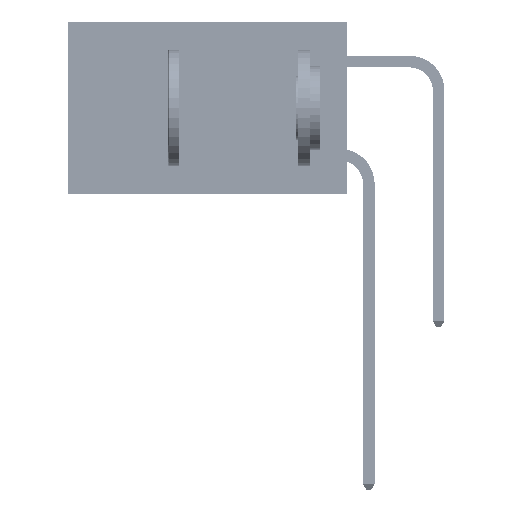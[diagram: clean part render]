
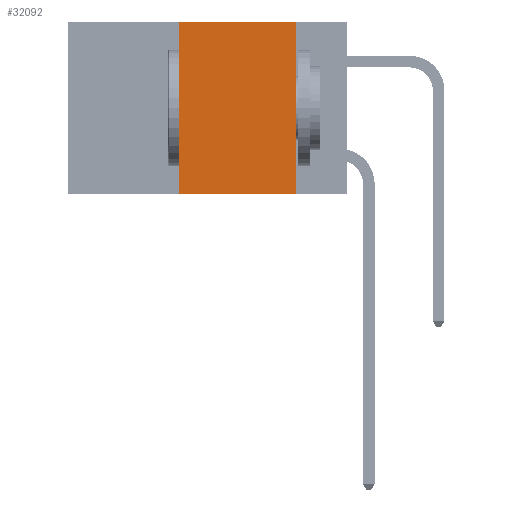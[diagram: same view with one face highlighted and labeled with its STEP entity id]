
A CAD part, left-side view. The second image highlights one B-rep face of the part: STEP entity #32092.
In plain terms, the highlighted planar face has unit normal (-1, 0, 0).
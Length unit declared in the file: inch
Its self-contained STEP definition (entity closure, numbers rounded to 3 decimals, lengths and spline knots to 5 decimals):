
#1645 = VECTOR ( 'NONE', #6929, 39.37008 ) ;
#2137 = VECTOR ( 'NONE', #41576, 39.37008 ) ;
#3097 = CARTESIAN_POINT ( 'NONE',  ( 0., 0.6, -0.37 ) ) ;
#4452 = CARTESIAN_POINT ( 'NONE',  ( 0., 0.36, 0. ) ) ;
#5223 = DIRECTION ( 'NONE',  ( 1., 0., 0. ) ) ;
#5965 = LINE ( 'NONE', #3097, #1645 ) ;
#5985 = FACE_OUTER_BOUND ( 'NONE', #19654, .T. ) ;
#6929 = DIRECTION ( 'NONE',  ( 0., -1., 0. ) ) ;
#8430 = ORIENTED_EDGE ( 'NONE', *, *, #25015, .F. ) ;
#9335 = CARTESIAN_POINT ( 'NONE',  ( 0., 0.36, -0.37 ) ) ;
#11548 = DIRECTION ( 'NONE',  ( 0., 0., 1. ) ) ;
#15015 = VERTEX_POINT ( 'NONE', #35116 ) ;
#15660 = VERTEX_POINT ( 'NONE', #4452 ) ;
#18143 = CARTESIAN_POINT ( 'NONE',  ( 0., 0.6, 0. ) ) ;
#19641 = LINE ( 'NONE', #46575, #25126 ) ;
#19654 = EDGE_LOOP ( 'NONE', ( #27246, #41443, #8430, #20321 ) ) ;
#19700 = VERTEX_POINT ( 'NONE', #9335 ) ;
#20321 = ORIENTED_EDGE ( 'NONE', *, *, #40414, .T. ) ;
#25015 = EDGE_CURVE ( 'NONE', #19700, #15660, #38855, .T. ) ;
#25126 = VECTOR ( 'NONE', #50342, 39.37008 ) ;
#26313 = AXIS2_PLACEMENT_3D ( 'NONE', #40685, #5223, #48464 ) ;
#26778 = LINE ( 'NONE', #18143, #2137 ) ;
#27246 = ORIENTED_EDGE ( 'NONE', *, *, #39658, .F. ) ;
#27627 = CARTESIAN_POINT ( 'NONE',  ( 0., 0.11, 0. ) ) ;
#27698 = VECTOR ( 'NONE', #11548, 39.37008 ) ;
#32092 = ADVANCED_FACE ( 'NONE', ( #5985 ), #48291, .F. ) ;
#35116 = CARTESIAN_POINT ( 'NONE',  ( 0., 0.11, -0.37 ) ) ;
#38855 = LINE ( 'NONE', #42873, #27698 ) ;
#39658 = EDGE_CURVE ( 'NONE', #41369, #15015, #19641, .T. ) ;
#40414 = EDGE_CURVE ( 'NONE', #19700, #15015, #5965, .T. ) ;
#40685 = CARTESIAN_POINT ( 'NONE',  ( 0., 0.6, 0. ) ) ;
#41369 = VERTEX_POINT ( 'NONE', #27627 ) ;
#41443 = ORIENTED_EDGE ( 'NONE', *, *, #41633, .F. ) ;
#41576 = DIRECTION ( 'NONE',  ( 0., -1., 0. ) ) ;
#41633 = EDGE_CURVE ( 'NONE', #15660, #41369, #26778, .T. ) ;
#42873 = CARTESIAN_POINT ( 'NONE',  ( 0., 0.36, 0. ) ) ;
#46575 = CARTESIAN_POINT ( 'NONE',  ( 0., 0.11, 0. ) ) ;
#48291 = PLANE ( 'NONE',  #26313 ) ;
#48464 = DIRECTION ( 'NONE',  ( 0., 0., -1. ) ) ;
#50342 = DIRECTION ( 'NONE',  ( 0., 0., -1. ) ) ;
